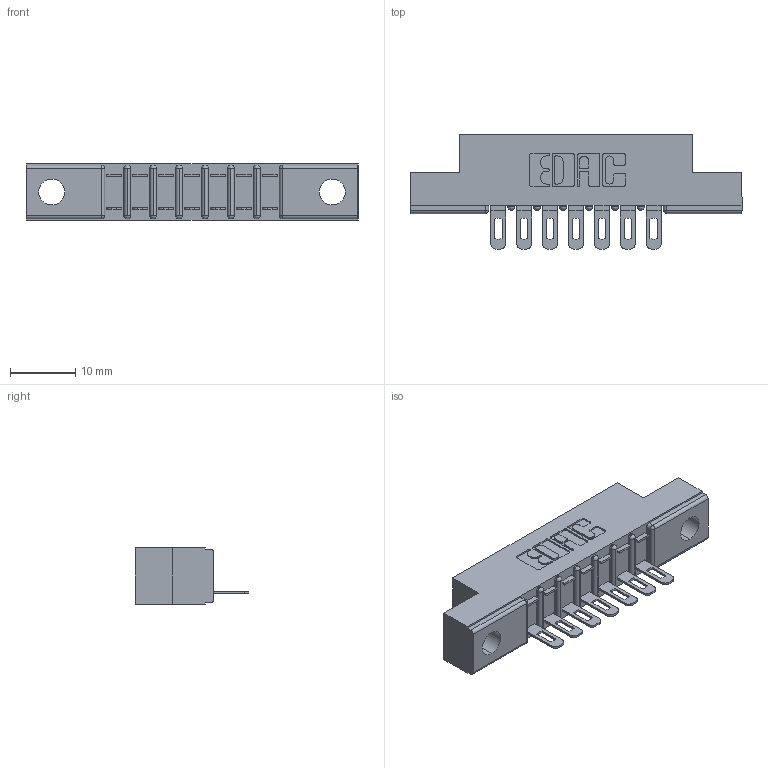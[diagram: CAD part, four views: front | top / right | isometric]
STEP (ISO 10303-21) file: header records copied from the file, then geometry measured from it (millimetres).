
FILE_DESCRIPTION (( 'STEP AP203' ), '1' );
FILE_NAME ('307-007-501-104.STEP', '2019-09-04T18:03:21', ( '' ), ( '' ), 'SwSTEP 2.0', 'SolidWorks 2016', '' );
FILE_SCHEMA (( 'CONFIG_CONTROL_DESIGN' ));
Length unit declared in the file: inch
Products named in the file (3): 307-007-501-104; 307-290-002_501; 307 Part_.156 Dia Mounting Holes
Assembly tree (8 placements, depth 2):
  307-007-501-104
    307 Part_.156 Dia Mounting Holes
    307-290-002_501  x7
Bounding box: 50.75 x 17.42 x 8.71 mm (x, y, z)
Volume: 3242.7 mm3; surface area: 5001.7 mm2
Topology: 8 solids, 8 shells, 672 faces, 2025 edges, 1326 vertices
Faces by surface type: plane 392, cylinder 264, sphere 16
Entity records: 11528 total; most frequent: CARTESIAN_POINT 1942, ORIENTED_EDGE 1930, DIRECTION 1899, EDGE_CURVE 965, LINE 725, VECTOR 725, VERTEX_POINT 630, AXIS2_PLACEMENT_3D 587
